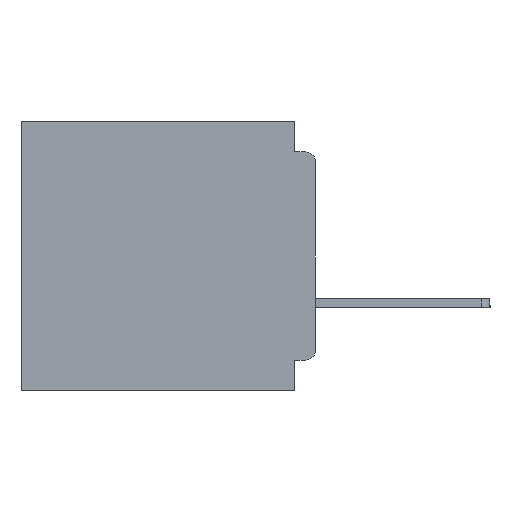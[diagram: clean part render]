
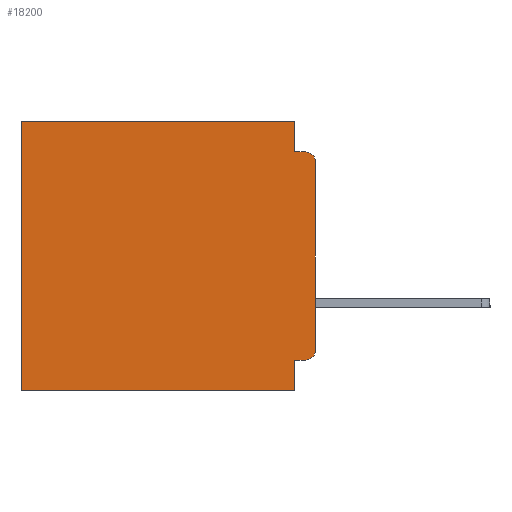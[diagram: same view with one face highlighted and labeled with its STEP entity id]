
A CAD part, left-side view. The second image highlights one B-rep face of the part: STEP entity #18200.
In plain terms, the highlighted planar face has unit normal (-1, 0, 0).
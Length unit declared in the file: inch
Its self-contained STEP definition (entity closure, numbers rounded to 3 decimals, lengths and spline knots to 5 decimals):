
#124 = AXIS2_PLACEMENT_3D ( 'NONE', #23042, #5126, #26065 ) ;
#151 = EDGE_CURVE ( 'NONE', #29736, #18512, #4091, .T. ) ;
#332 = VECTOR ( 'NONE', #26664, 39.37008 ) ;
#905 = CARTESIAN_POINT ( 'NONE',  ( 0.3, 0.015, -0.06 ) ) ;
#1349 = VERTEX_POINT ( 'NONE', #13569 ) ;
#1927 = LINE ( 'NONE', #33061, #32880 ) ;
#2260 = LINE ( 'NONE', #7539, #9316 ) ;
#2699 = CARTESIAN_POINT ( 'NONE',  ( 0.3, 0., -0.4 ) ) ;
#2788 = CARTESIAN_POINT ( 'NONE',  ( 0.3, 0., -0.4 ) ) ;
#2806 = VECTOR ( 'NONE', #30486, 39.37008 ) ;
#2807 = CARTESIAN_POINT ( 'NONE',  ( 0.3, 0., -0.06 ) ) ;
#3302 = CARTESIAN_POINT ( 'NONE',  ( 0.3, 0., -0.045 ) ) ;
#3759 = CARTESIAN_POINT ( 'NONE',  ( 0.3, 0.015, -0.355 ) ) ;
#4091 = CIRCLE ( 'NONE', #24497, 0.015 ) ;
#4092 = CARTESIAN_POINT ( 'NONE',  ( 0.3, 0.031, -0.4 ) ) ;
#4112 = LINE ( 'NONE', #3302, #34071 ) ;
#4129 = ORIENTED_EDGE ( 'NONE', *, *, #151, .T. ) ;
#4261 = VERTEX_POINT ( 'NONE', #4092 ) ;
#4453 = ORIENTED_EDGE ( 'NONE', *, *, #17598, .F. ) ;
#5126 = DIRECTION ( 'NONE',  ( -1., 0., 0. ) ) ;
#5615 = DIRECTION ( 'NONE',  ( 0., 0., -1. ) ) ;
#5785 = DIRECTION ( 'NONE',  ( 0., 0., -1. ) ) ;
#6352 = DIRECTION ( 'NONE',  ( 0., -1., 0. ) ) ;
#6538 = CARTESIAN_POINT ( 'NONE',  ( 0.3, 0.031, -0.4 ) ) ;
#6550 = ORIENTED_EDGE ( 'NONE', *, *, #19963, .T. ) ;
#6985 = ORIENTED_EDGE ( 'NONE', *, *, #27127, .F. ) ;
#7539 = CARTESIAN_POINT ( 'NONE',  ( 0.3, 0.031, 0. ) ) ;
#8244 = CARTESIAN_POINT ( 'NONE',  ( 0.3, 0., 0. ) ) ;
#8556 = EDGE_LOOP ( 'NONE', ( #37794, #4129, #34345, #34902, #24159, #6550, #4453, #24985, #6985, #15506 ) ) ;
#8657 = CARTESIAN_POINT ( 'NONE',  ( 0.3, 0., -0.4 ) ) ;
#8707 = DIRECTION ( 'NONE',  ( 0., 1., 0. ) ) ;
#8985 = EDGE_CURVE ( 'NONE', #1349, #15303, #2260, .T. ) ;
#9316 = VECTOR ( 'NONE', #10512, 39.37008 ) ;
#10512 = DIRECTION ( 'NONE',  ( 0., 0., -1. ) ) ;
#10545 = LINE ( 'NONE', #21042, #25525 ) ;
#12106 = DIRECTION ( 'NONE',  ( 0., 1., 0. ) ) ;
#12246 = VERTEX_POINT ( 'NONE', #24094 ) ;
#12659 = LINE ( 'NONE', #6538, #2806 ) ;
#13569 = CARTESIAN_POINT ( 'NONE',  ( 0.3, 0.031, 0. ) ) ;
#14043 = CARTESIAN_POINT ( 'NONE',  ( 0.3, 0., -0.34 ) ) ;
#14737 = EDGE_CURVE ( 'NONE', #29736, #25722, #24251, .T. ) ;
#15303 = VERTEX_POINT ( 'NONE', #20321 ) ;
#15405 = LINE ( 'NONE', #8244, #38208 ) ;
#15506 = ORIENTED_EDGE ( 'NONE', *, *, #19104, .T. ) ;
#15638 = FACE_OUTER_BOUND ( 'NONE', #8556, .T. ) ;
#16170 = VECTOR ( 'NONE', #8707, 39.37008 ) ;
#16249 = CARTESIAN_POINT ( 'NONE',  ( 0.3, 0.015, -0.045 ) ) ;
#17598 = EDGE_CURVE ( 'NONE', #4261, #12246, #22212, .T. ) ;
#18200 = ADVANCED_FACE ( 'NONE', ( #15638 ), #20678, .F. ) ;
#18512 = VERTEX_POINT ( 'NONE', #16249 ) ;
#18836 = EDGE_CURVE ( 'NONE', #15303, #18512, #4112, .T. ) ;
#19104 = EDGE_CURVE ( 'NONE', #35521, #25722, #26558, .T. ) ;
#19963 = EDGE_CURVE ( 'NONE', #36151, #12246, #10545, .T. ) ;
#20321 = CARTESIAN_POINT ( 'NONE',  ( 0.3, 0.031, -0.045 ) ) ;
#20678 = PLANE ( 'NONE',  #33280 ) ;
#21042 = CARTESIAN_POINT ( 'NONE',  ( 0.3, 0.437, -0.4 ) ) ;
#22212 = LINE ( 'NONE', #2788, #16170 ) ;
#23042 = CARTESIAN_POINT ( 'NONE',  ( 0.3, 0.015, -0.34 ) ) ;
#23671 = DIRECTION ( 'NONE',  ( 1., 0., 0. ) ) ;
#24022 = DIRECTION ( 'NONE',  ( 0., 0., -1. ) ) ;
#24094 = CARTESIAN_POINT ( 'NONE',  ( 0.3, 0.437, -0.4 ) ) ;
#24159 = ORIENTED_EDGE ( 'NONE', *, *, #29145, .T. ) ;
#24251 = LINE ( 'NONE', #2699, #332 ) ;
#24497 = AXIS2_PLACEMENT_3D ( 'NONE', #905, #24669, #5615 ) ;
#24669 = DIRECTION ( 'NONE',  ( -1., 0., 0. ) ) ;
#24985 = ORIENTED_EDGE ( 'NONE', *, *, #35470, .F. ) ;
#25097 = CARTESIAN_POINT ( 'NONE',  ( 0.3, 0.437, 0. ) ) ;
#25525 = VECTOR ( 'NONE', #24022, 39.37008 ) ;
#25722 = VERTEX_POINT ( 'NONE', #14043 ) ;
#26065 = DIRECTION ( 'NONE',  ( 0., 0., -1. ) ) ;
#26558 = CIRCLE ( 'NONE', #124, 0.015 ) ;
#26664 = DIRECTION ( 'NONE',  ( 0., 0., -1. ) ) ;
#27127 = EDGE_CURVE ( 'NONE', #35521, #30646, #1927, .T. ) ;
#29145 = EDGE_CURVE ( 'NONE', #1349, #36151, #15405, .T. ) ;
#29208 = DIRECTION ( 'NONE',  ( 0., 1., 0. ) ) ;
#29736 = VERTEX_POINT ( 'NONE', #2807 ) ;
#30486 = DIRECTION ( 'NONE',  ( 0., 0., -1. ) ) ;
#30646 = VERTEX_POINT ( 'NONE', #34965 ) ;
#32880 = VECTOR ( 'NONE', #12106, 39.37008 ) ;
#33061 = CARTESIAN_POINT ( 'NONE',  ( 0.3, 0., -0.355 ) ) ;
#33280 = AXIS2_PLACEMENT_3D ( 'NONE', #8657, #23671, #5785 ) ;
#34071 = VECTOR ( 'NONE', #6352, 39.37008 ) ;
#34345 = ORIENTED_EDGE ( 'NONE', *, *, #18836, .F. ) ;
#34902 = ORIENTED_EDGE ( 'NONE', *, *, #8985, .F. ) ;
#34965 = CARTESIAN_POINT ( 'NONE',  ( 0.3, 0.031, -0.355 ) ) ;
#35470 = EDGE_CURVE ( 'NONE', #30646, #4261, #12659, .T. ) ;
#35521 = VERTEX_POINT ( 'NONE', #3759 ) ;
#36151 = VERTEX_POINT ( 'NONE', #25097 ) ;
#37794 = ORIENTED_EDGE ( 'NONE', *, *, #14737, .F. ) ;
#38208 = VECTOR ( 'NONE', #29208, 39.37008 ) ;
